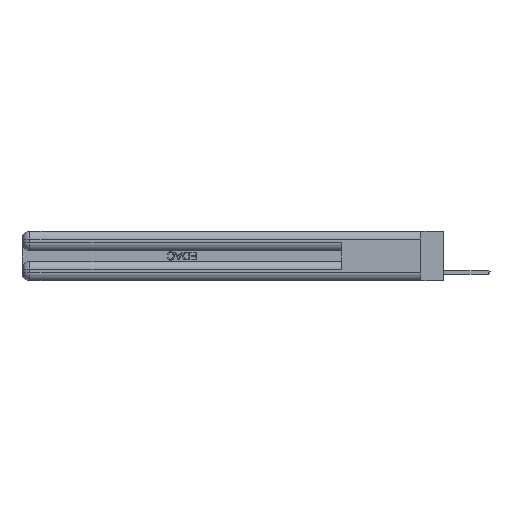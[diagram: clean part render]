
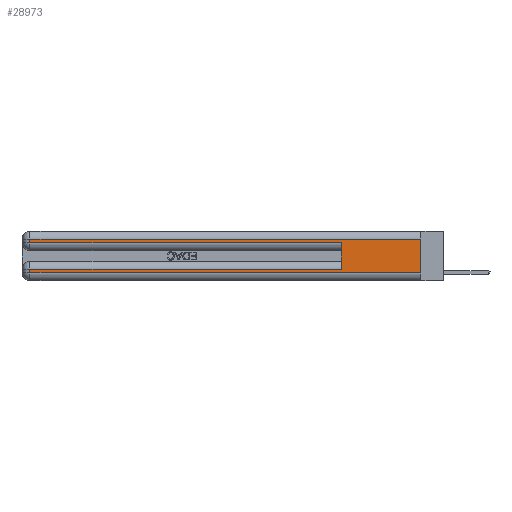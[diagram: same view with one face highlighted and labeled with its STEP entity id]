
A CAD part, left-side view. The second image highlights one B-rep face of the part: STEP entity #28973.
In plain terms, the highlighted planar face has unit normal (-1, 0, 0).
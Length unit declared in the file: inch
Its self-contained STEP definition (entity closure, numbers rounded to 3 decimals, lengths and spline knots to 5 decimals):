
#852 = AXIS2_PLACEMENT_3D ( 'NONE', #27834, #25161, #33010 ) ;
#887 = DIRECTION ( 'NONE',  ( 0., 0., -1. ) ) ;
#1310 = DIRECTION ( 'NONE',  ( 0., -1., 0. ) ) ;
#2077 = VECTOR ( 'NONE', #5509, 39.37008 ) ;
#3059 = PLANE ( 'NONE',  #852 ) ;
#3253 = VECTOR ( 'NONE', #24934, 39.37008 ) ;
#4162 = CARTESIAN_POINT ( 'NONE',  ( 0., 0., 0.06 ) ) ;
#4889 = DIRECTION ( 'NONE',  ( 0., 1., 0. ) ) ;
#5421 = VECTOR ( 'NONE', #4889, 39.37008 ) ;
#5509 = DIRECTION ( 'NONE',  ( 0., 1., 0. ) ) ;
#5916 = FACE_OUTER_BOUND ( 'NONE', #27453, .T. ) ;
#6492 = DIRECTION ( 'NONE',  ( 0., -1., 0. ) ) ;
#7572 = EDGE_CURVE ( 'NONE', #10580, #20965, #21451, .T. ) ;
#8594 = EDGE_CURVE ( 'NONE', #22502, #19942, #29933, .T. ) ;
#9071 = LINE ( 'NONE', #17275, #3253 ) ;
#9121 = CARTESIAN_POINT ( 'NONE',  ( 0., 0.6, 0.145 ) ) ;
#9460 = ORIENTED_EDGE ( 'NONE', *, *, #23893, .T. ) ;
#10125 = ORIENTED_EDGE ( 'NONE', *, *, #31348, .T. ) ;
#10357 = LINE ( 'NONE', #4162, #19766 ) ;
#10580 = VERTEX_POINT ( 'NONE', #28177 ) ;
#10807 = VERTEX_POINT ( 'NONE', #12469 ) ;
#11038 = CARTESIAN_POINT ( 'NONE',  ( 0., 0., 0.085 ) ) ;
#11587 = LINE ( 'NONE', #25317, #15265 ) ;
#12469 = CARTESIAN_POINT ( 'NONE',  ( 0., 2.94, 0.285 ) ) ;
#13001 = EDGE_CURVE ( 'NONE', #10807, #27873, #17008, .T. ) ;
#15265 = VECTOR ( 'NONE', #887, 39.37008 ) ;
#16368 = VERTEX_POINT ( 'NONE', #21892 ) ;
#16401 = DIRECTION ( 'NONE',  ( 0., 0., -1. ) ) ;
#17008 = LINE ( 'NONE', #27886, #19916 ) ;
#17275 = CARTESIAN_POINT ( 'NONE',  ( 0., 2.94, 0.37 ) ) ;
#17450 = VECTOR ( 'NONE', #16401, 39.37008 ) ;
#18047 = ORIENTED_EDGE ( 'NONE', *, *, #20773, .T. ) ;
#18921 = LINE ( 'NONE', #19265, #17450 ) ;
#19134 = ORIENTED_EDGE ( 'NONE', *, *, #8594, .T. ) ;
#19265 = CARTESIAN_POINT ( 'NONE',  ( 0., 0., 0.37 ) ) ;
#19301 = ORIENTED_EDGE ( 'NONE', *, *, #13001, .T. ) ;
#19371 = EDGE_CURVE ( 'NONE', #10580, #26596, #18921, .T. ) ;
#19766 = VECTOR ( 'NONE', #1310, 39.37008 ) ;
#19916 = VECTOR ( 'NONE', #6492, 39.37008 ) ;
#19942 = VERTEX_POINT ( 'NONE', #33430 ) ;
#20773 = EDGE_CURVE ( 'NONE', #19942, #16368, #11587, .T. ) ;
#20796 = CARTESIAN_POINT ( 'NONE',  ( 0., 0., 0.06 ) ) ;
#20965 = VERTEX_POINT ( 'NONE', #28681 ) ;
#21451 = LINE ( 'NONE', #29841, #5421 ) ;
#21892 = CARTESIAN_POINT ( 'NONE',  ( 0., 2.94, 0.06 ) ) ;
#22179 = ORIENTED_EDGE ( 'NONE', *, *, #34648, .F. ) ;
#22502 = VERTEX_POINT ( 'NONE', #24583 ) ;
#23893 = EDGE_CURVE ( 'NONE', #20965, #10807, #9071, .T. ) ;
#24583 = CARTESIAN_POINT ( 'NONE',  ( 0., 0.6, 0.085 ) ) ;
#24690 = ORIENTED_EDGE ( 'NONE', *, *, #19371, .F. ) ;
#24934 = DIRECTION ( 'NONE',  ( 0., 0., -1. ) ) ;
#25161 = DIRECTION ( 'NONE',  ( 1., 0., 0. ) ) ;
#25238 = ORIENTED_EDGE ( 'NONE', *, *, #7572, .T. ) ;
#25317 = CARTESIAN_POINT ( 'NONE',  ( 0., 2.94, 0.37 ) ) ;
#26596 = VERTEX_POINT ( 'NONE', #20796 ) ;
#27453 = EDGE_LOOP ( 'NONE', ( #24690, #25238, #9460, #19301, #22179, #19134, #18047, #10125 ) ) ;
#27834 = CARTESIAN_POINT ( 'NONE',  ( 0., 0., 0.37 ) ) ;
#27873 = VERTEX_POINT ( 'NONE', #31493 ) ;
#27886 = CARTESIAN_POINT ( 'NONE',  ( 0., 0., 0.285 ) ) ;
#28177 = CARTESIAN_POINT ( 'NONE',  ( 0., 0., 0.31 ) ) ;
#28681 = CARTESIAN_POINT ( 'NONE',  ( 0., 2.94, 0.31 ) ) ;
#28973 = ADVANCED_FACE ( 'NONE', ( #5916 ), #3059, .F. ) ;
#29841 = CARTESIAN_POINT ( 'NONE',  ( 0., 0., 0.31 ) ) ;
#29933 = LINE ( 'NONE', #11038, #2077 ) ;
#30681 = LINE ( 'NONE', #9121, #34638 ) ;
#31348 = EDGE_CURVE ( 'NONE', #16368, #26596, #10357, .T. ) ;
#31493 = CARTESIAN_POINT ( 'NONE',  ( 0., 0.6, 0.285 ) ) ;
#33010 = DIRECTION ( 'NONE',  ( 0., 0., -1. ) ) ;
#33430 = CARTESIAN_POINT ( 'NONE',  ( 0., 2.94, 0.085 ) ) ;
#33544 = DIRECTION ( 'NONE',  ( 0., 0., 1. ) ) ;
#34638 = VECTOR ( 'NONE', #33544, 39.37008 ) ;
#34648 = EDGE_CURVE ( 'NONE', #22502, #27873, #30681, .T. ) ;
